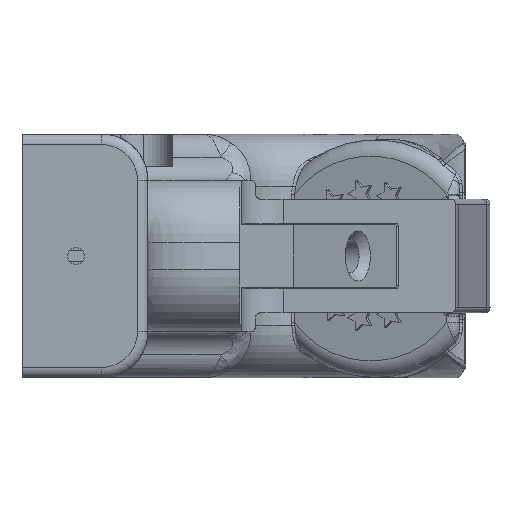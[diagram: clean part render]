
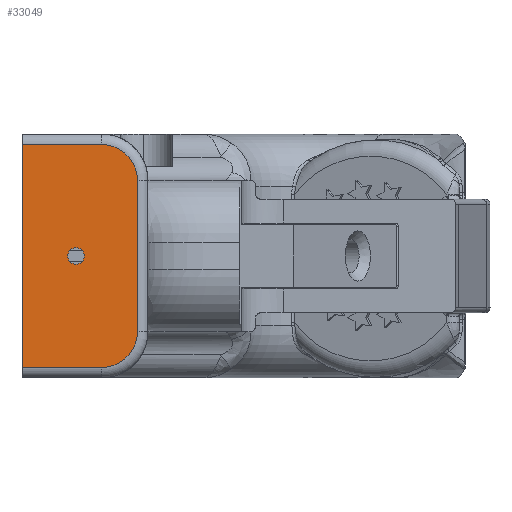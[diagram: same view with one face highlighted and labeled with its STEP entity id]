
A CAD part, left-side view. The second image highlights one B-rep face of the part: STEP entity #33049.
In plain terms, the highlighted planar face has unit normal (-1, 0, 0).
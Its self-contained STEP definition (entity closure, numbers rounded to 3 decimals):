
#3001=LINE('',#48776,#6525);
#4338=LINE('',#62567,#7862);
#4415=LINE('',#63559,#7939);
#4416=LINE('',#63560,#7940);
#6525=VECTOR('',#38390,33.958);
#7862=VECTOR('',#41493,23.019);
#7939=VECTOR('',#41856,12.12);
#7940=VECTOR('',#41857,12.12);
#9234=PLANE('',#34850);
#9448=FACE_BOUND('',#12921,.T.);
#11066=FACE_OUTER_BOUND('',#12920,.T.);
#12920=EDGE_LOOP('',(#29308,#29309,#29310,#29311,#29312,#29313));
#12921=EDGE_LOOP('',(#29314));
#13234=CIRCLE('',#34705,1.25);
#13237=CIRCLE('',#34710,5.47);
#13241=CIRCLE('',#34722,5.47);
#14934=VERTEX_POINT('',#48773);
#14935=VERTEX_POINT('',#48775);
#16112=VERTEX_POINT('',#62561);
#16113=VERTEX_POINT('',#62564);
#16114=VERTEX_POINT('',#62566);
#16115=VERTEX_POINT('',#62570);
#16124=VERTEX_POINT('',#62596);
#18563=EDGE_CURVE('',#14935,#14934,#3001,.T.);
#20435=EDGE_CURVE('',#16112,#16112,#13234,.T.);
#20437=EDGE_CURVE('',#16113,#16114,#4338,.T.);
#20439=EDGE_CURVE('',#16114,#16115,#13237,.T.);
#20453=EDGE_CURVE('',#16124,#16113,#13241,.T.);
#20602=EDGE_CURVE('',#14935,#16124,#4415,.T.);
#20603=EDGE_CURVE('',#16115,#14934,#4416,.T.);
#29308=ORIENTED_EDGE('',*,*,#20602,.F.);
#29309=ORIENTED_EDGE('',*,*,#18563,.T.);
#29310=ORIENTED_EDGE('',*,*,#20603,.F.);
#29311=ORIENTED_EDGE('',*,*,#20439,.F.);
#29312=ORIENTED_EDGE('',*,*,#20437,.F.);
#29313=ORIENTED_EDGE('',*,*,#20453,.F.);
#29314=ORIENTED_EDGE('',*,*,#20435,.T.);
#33049=ADVANCED_FACE('',(#11066,#9448),#9234,.T.);
#34705=AXIS2_PLACEMENT_3D('',#62562,#41487,#41488);
#34710=AXIS2_PLACEMENT_3D('',#62571,#41498,#41499);
#34722=AXIS2_PLACEMENT_3D('',#62598,#41528,#41529);
#34850=AXIS2_PLACEMENT_3D('',#63558,#41854,#41855);
#38390=DIRECTION('',(0.,0.,-1.));
#41487=DIRECTION('center_axis',(1.,0.,0.));
#41488=DIRECTION('ref_axis',(0.,0.,
-1.));
#41493=DIRECTION('',(0.,0.,-1.));
#41498=DIRECTION('center_axis',(1.,0.,0.));
#41499=DIRECTION('ref_axis',(0.,-0.707,-0.707));
#41528=DIRECTION('center_axis',(1.,0.,0.));
#41529=DIRECTION('ref_axis',(0.,-0.707,0.707));
#41854=DIRECTION('center_axis',(-1.,0.,0.));
#41855=DIRECTION('ref_axis',(0.,0.,
1.));
#41856=DIRECTION('',(0.,-1.,0.));
#41857=DIRECTION('',(0.,1.,0.));
#48773=CARTESIAN_POINT('',(-191.173,5.586,-16.979));
#48775=CARTESIAN_POINT('',(-191.173,5.586,16.979));
#48776=CARTESIAN_POINT('',(-191.173,5.586,-17.583));
#62561=CARTESIAN_POINT('',(-191.173,-2.633,1.25));
#62562=CARTESIAN_POINT('Origin',(-191.173,-2.633,0.));
#62564=CARTESIAN_POINT('',(-191.173,-12.004,11.509));
#62566=CARTESIAN_POINT('',(-191.173,-12.004,-11.509));
#62567=CARTESIAN_POINT('',(-191.173,-12.004,-11.509));
#62570=CARTESIAN_POINT('',(-191.173,-6.534,-16.979));
#62571=CARTESIAN_POINT('Origin',(-191.173,-6.534,-11.509));
#62596=CARTESIAN_POINT('',(-191.173,-6.534,16.979));
#62598=CARTESIAN_POINT('Origin',(-191.173,-6.534,11.509));
#63558=CARTESIAN_POINT('Origin',(-191.173,-0.777,-11.509));
#63559=CARTESIAN_POINT('',(-191.173,2.405,16.979));
#63560=CARTESIAN_POINT('',(-191.173,2.405,-16.979));
